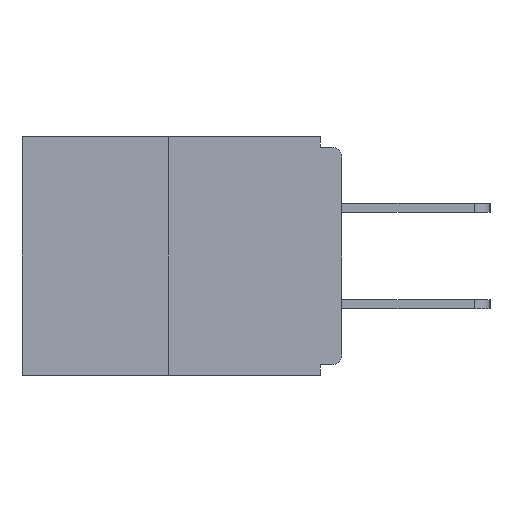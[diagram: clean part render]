
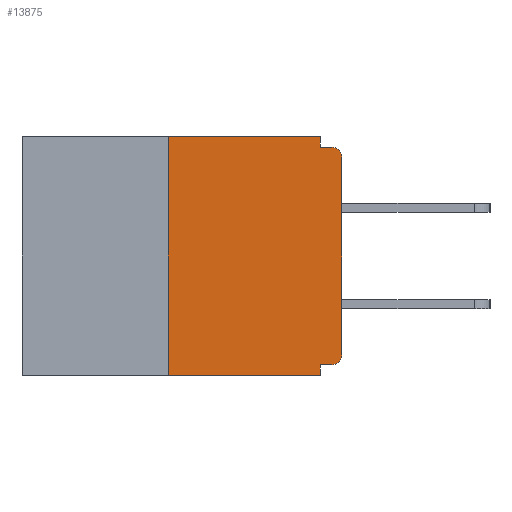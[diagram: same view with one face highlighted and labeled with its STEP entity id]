
A CAD part, left-side view. The second image highlights one B-rep face of the part: STEP entity #13875.
In plain terms, the highlighted planar face has unit normal (-1, 0, 0).
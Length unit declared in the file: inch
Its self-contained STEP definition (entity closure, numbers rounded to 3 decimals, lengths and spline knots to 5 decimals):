
#11 = EDGE_CURVE ( 'NONE', #25252, #26242, #4622, .T. ) ;
#834 = VERTEX_POINT ( 'NONE', #9572 ) ;
#1296 = LINE ( 'NONE', #1832, #19520 ) ;
#1495 = VERTEX_POINT ( 'NONE', #21342 ) ;
#1832 = CARTESIAN_POINT ( 'NONE',  ( 0., 0.25, 0. ) ) ;
#2031 = VERTEX_POINT ( 'NONE', #5335 ) ;
#2564 = CARTESIAN_POINT ( 'NONE',  ( 0., 0., 0. ) ) ;
#2932 = ORIENTED_EDGE ( 'NONE', *, *, #9587, .F. ) ;
#2956 = CARTESIAN_POINT ( 'NONE',  ( 0., 0.25, -0.343 ) ) ;
#3024 = DIRECTION ( 'NONE',  ( 0., 0., -1. ) ) ;
#3543 = CARTESIAN_POINT ( 'NONE',  ( 0., 0.25, 0. ) ) ;
#3791 = DIRECTION ( 'NONE',  ( -1., 0., 0. ) ) ;
#3941 = DIRECTION ( 'NONE',  ( 0., 0., -1. ) ) ;
#4580 = ORIENTED_EDGE ( 'NONE', *, *, #16303, .T. ) ;
#4622 = LINE ( 'NONE', #6640, #6468 ) ;
#5009 = ORIENTED_EDGE ( 'NONE', *, *, #5932, .F. ) ;
#5310 = CIRCLE ( 'NONE', #23774, 0.015 ) ;
#5335 = CARTESIAN_POINT ( 'NONE',  ( 0., 0.031, 0. ) ) ;
#5657 = ORIENTED_EDGE ( 'NONE', *, *, #17982, .F. ) ;
#5743 = VERTEX_POINT ( 'NONE', #16746 ) ;
#5932 = EDGE_CURVE ( 'NONE', #2031, #5743, #11617, .T. ) ;
#5959 = VECTOR ( 'NONE', #3024, 39.37008 ) ;
#6434 = CARTESIAN_POINT ( 'NONE',  ( 0., 0.031, -0.343 ) ) ;
#6468 = VECTOR ( 'NONE', #7039, 39.37008 ) ;
#6640 = CARTESIAN_POINT ( 'NONE',  ( 0., 0., -0.328 ) ) ;
#6648 = VECTOR ( 'NONE', #23576, 39.37008 ) ;
#6706 = LINE ( 'NONE', #2564, #24176 ) ;
#6910 = LINE ( 'NONE', #15115, #5959 ) ;
#7039 = DIRECTION ( 'NONE',  ( 0., 1., 0. ) ) ;
#7735 = EDGE_LOOP ( 'NONE', ( #2932, #18758, #10124, #9924, #9598, #8878, #4580, #12253, #5657, #5009 ) ) ;
#8219 = CARTESIAN_POINT ( 'NONE',  ( 0., 0.015, -0.313 ) ) ;
#8323 = DIRECTION ( 'NONE',  ( 0., 0., 1. ) ) ;
#8878 = ORIENTED_EDGE ( 'NONE', *, *, #15665, .T. ) ;
#8983 = CARTESIAN_POINT ( 'NONE',  ( 0., 0., -0.313 ) ) ;
#9041 = VECTOR ( 'NONE', #20946, 39.37008 ) ;
#9326 = CARTESIAN_POINT ( 'NONE',  ( 0., 0.46, -0.343 ) ) ;
#9451 = LINE ( 'NONE', #9326, #18575 ) ;
#9572 = CARTESIAN_POINT ( 'NONE',  ( 0., 0., -0.03 ) ) ;
#9587 = EDGE_CURVE ( 'NONE', #13793, #2031, #16787, .T. ) ;
#9598 = ORIENTED_EDGE ( 'NONE', *, *, #11, .F. ) ;
#9924 = ORIENTED_EDGE ( 'NONE', *, *, #21686, .F. ) ;
#10124 = ORIENTED_EDGE ( 'NONE', *, *, #11197, .T. ) ;
#10366 = PLANE ( 'NONE',  #11766 ) ;
#11191 = CARTESIAN_POINT ( 'NONE',  ( 0., 0., -0.015 ) ) ;
#11197 = EDGE_CURVE ( 'NONE', #21308, #16412, #9451, .T. ) ;
#11617 = LINE ( 'NONE', #17802, #23229 ) ;
#11734 = DIRECTION ( 'NONE',  ( 0., 0., -1. ) ) ;
#11766 = AXIS2_PLACEMENT_3D ( 'NONE', #20978, #16557, #18570 ) ;
#11997 = CARTESIAN_POINT ( 'NONE',  ( 0., 0.031, -0.328 ) ) ;
#12253 = ORIENTED_EDGE ( 'NONE', *, *, #13808, .T. ) ;
#13403 = AXIS2_PLACEMENT_3D ( 'NONE', #8219, #18579, #3941 ) ;
#13793 = VERTEX_POINT ( 'NONE', #3543 ) ;
#13808 = EDGE_CURVE ( 'NONE', #834, #1495, #5310, .T. ) ;
#13875 = ADVANCED_FACE ( 'NONE', ( #24757 ), #10366, .F. ) ;
#14000 = CARTESIAN_POINT ( 'NONE',  ( 0., 0.015, -0.03 ) ) ;
#14175 = DIRECTION ( 'NONE',  ( 0., 0., 1. ) ) ;
#14260 = CIRCLE ( 'NONE', #13403, 0.015 ) ;
#15006 = EDGE_CURVE ( 'NONE', #21308, #13793, #1296, .T. ) ;
#15115 = CARTESIAN_POINT ( 'NONE',  ( 0., 0.031, -0.343 ) ) ;
#15355 = LINE ( 'NONE', #11191, #6648 ) ;
#15665 = EDGE_CURVE ( 'NONE', #25252, #23816, #14260, .T. ) ;
#16303 = EDGE_CURVE ( 'NONE', #23816, #834, #6706, .T. ) ;
#16412 = VERTEX_POINT ( 'NONE', #6434 ) ;
#16557 = DIRECTION ( 'NONE',  ( 1., 0., 0. ) ) ;
#16746 = CARTESIAN_POINT ( 'NONE',  ( 0., 0.031, -0.015 ) ) ;
#16787 = LINE ( 'NONE', #25245, #9041 ) ;
#17802 = CARTESIAN_POINT ( 'NONE',  ( 0., 0.031, 0. ) ) ;
#17982 = EDGE_CURVE ( 'NONE', #5743, #1495, #15355, .T. ) ;
#18570 = DIRECTION ( 'NONE',  ( 0., 0., -1. ) ) ;
#18575 = VECTOR ( 'NONE', #25742, 39.37008 ) ;
#18579 = DIRECTION ( 'NONE',  ( -1., 0., 0. ) ) ;
#18758 = ORIENTED_EDGE ( 'NONE', *, *, #15006, .F. ) ;
#19520 = VECTOR ( 'NONE', #14175, 39.37008 ) ;
#20946 = DIRECTION ( 'NONE',  ( 0., -1., 0. ) ) ;
#20978 = CARTESIAN_POINT ( 'NONE',  ( 0., 0.46, 0. ) ) ;
#21308 = VERTEX_POINT ( 'NONE', #2956 ) ;
#21342 = CARTESIAN_POINT ( 'NONE',  ( 0., 0.015, -0.015 ) ) ;
#21686 = EDGE_CURVE ( 'NONE', #26242, #16412, #6910, .T. ) ;
#23229 = VECTOR ( 'NONE', #26011, 39.37008 ) ;
#23576 = DIRECTION ( 'NONE',  ( 0., -1., 0. ) ) ;
#23774 = AXIS2_PLACEMENT_3D ( 'NONE', #14000, #3791, #11734 ) ;
#23816 = VERTEX_POINT ( 'NONE', #8983 ) ;
#24176 = VECTOR ( 'NONE', #8323, 39.37008 ) ;
#24757 = FACE_OUTER_BOUND ( 'NONE', #7735, .T. ) ;
#25245 = CARTESIAN_POINT ( 'NONE',  ( 0., 0.46, 0. ) ) ;
#25252 = VERTEX_POINT ( 'NONE', #25540 ) ;
#25540 = CARTESIAN_POINT ( 'NONE',  ( 0., 0.015, -0.328 ) ) ;
#25742 = DIRECTION ( 'NONE',  ( 0., -1., 0. ) ) ;
#26011 = DIRECTION ( 'NONE',  ( 0., 0., -1. ) ) ;
#26242 = VERTEX_POINT ( 'NONE', #11997 ) ;
